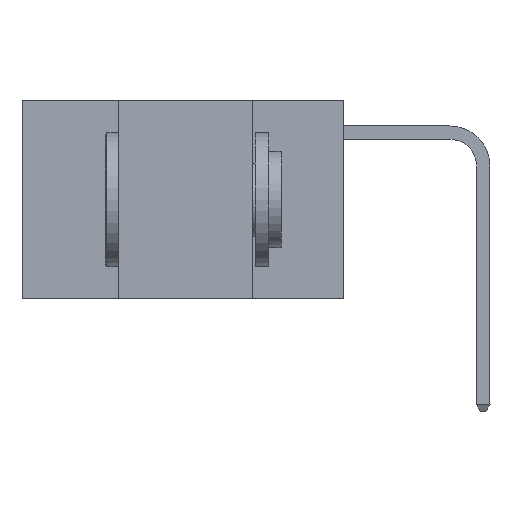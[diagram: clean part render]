
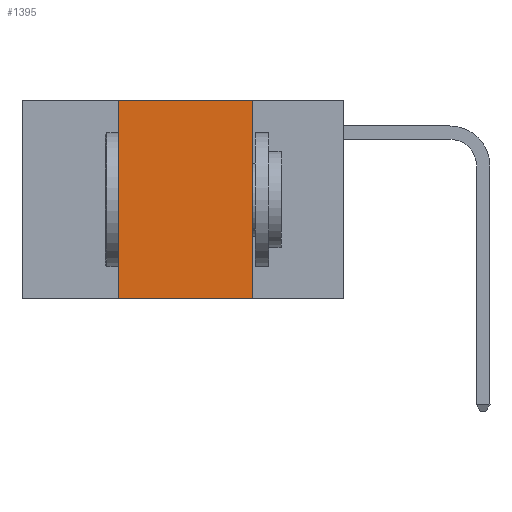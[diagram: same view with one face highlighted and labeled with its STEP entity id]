
A CAD part, left-side view. The second image highlights one B-rep face of the part: STEP entity #1395.
In plain terms, the highlighted planar face has unit normal (-1, 0, 0).
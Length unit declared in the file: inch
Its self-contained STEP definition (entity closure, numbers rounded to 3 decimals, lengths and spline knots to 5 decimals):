
#246 = CARTESIAN_POINT ( 'NONE',  ( 0., 0.42, -0.37 ) ) ;
#739 = ORIENTED_EDGE ( 'NONE', *, *, #8518, .F. ) ;
#756 = ORIENTED_EDGE ( 'NONE', *, *, #2793, .F. ) ;
#1099 = LINE ( 'NONE', #11558, #6491 ) ;
#1395 = ADVANCED_FACE ( 'NONE', ( #13389 ), #9598, .F. ) ;
#1751 = EDGE_LOOP ( 'NONE', ( #1821, #756, #739, #4710 ) ) ;
#1821 = ORIENTED_EDGE ( 'NONE', *, *, #4781, .F. ) ;
#2010 = DIRECTION ( 'NONE',  ( 1., 0., 0. ) ) ;
#2324 = DIRECTION ( 'NONE',  ( 0., 0., 1. ) ) ;
#2411 = VECTOR ( 'NONE', #10360, 39.37008 ) ;
#2793 = EDGE_CURVE ( 'NONE', #4568, #4338, #10934, .T. ) ;
#2833 = CARTESIAN_POINT ( 'NONE',  ( 0., 0.6, 0. ) ) ;
#3385 = VECTOR ( 'NONE', #2324, 39.37008 ) ;
#3481 = LINE ( 'NONE', #10780, #11895 ) ;
#4338 = VERTEX_POINT ( 'NONE', #7771 ) ;
#4568 = VERTEX_POINT ( 'NONE', #12615 ) ;
#4710 = ORIENTED_EDGE ( 'NONE', *, *, #5644, .T. ) ;
#4781 = EDGE_CURVE ( 'NONE', #4338, #8259, #3481, .T. ) ;
#5265 = DIRECTION ( 'NONE',  ( 0., 0., -1. ) ) ;
#5644 = EDGE_CURVE ( 'NONE', #7839, #8259, #1099, .T. ) ;
#6240 = LINE ( 'NONE', #7686, #3385 ) ;
#6491 = VECTOR ( 'NONE', #8222, 39.37008 ) ;
#7686 = CARTESIAN_POINT ( 'NONE',  ( 0., 0.42, 0. ) ) ;
#7771 = CARTESIAN_POINT ( 'NONE',  ( 0., 0.17, 0. ) ) ;
#7839 = VERTEX_POINT ( 'NONE', #246 ) ;
#8222 = DIRECTION ( 'NONE',  ( 0., -1., 0. ) ) ;
#8257 = AXIS2_PLACEMENT_3D ( 'NONE', #2833, #2010, #5265 ) ;
#8259 = VERTEX_POINT ( 'NONE', #10843 ) ;
#8518 = EDGE_CURVE ( 'NONE', #7839, #4568, #6240, .T. ) ;
#9598 = PLANE ( 'NONE',  #8257 ) ;
#10360 = DIRECTION ( 'NONE',  ( 0., -1., 0. ) ) ;
#10780 = CARTESIAN_POINT ( 'NONE',  ( 0., 0.17, 0. ) ) ;
#10843 = CARTESIAN_POINT ( 'NONE',  ( 0., 0.17, -0.37 ) ) ;
#10934 = LINE ( 'NONE', #11514, #2411 ) ;
#10956 = DIRECTION ( 'NONE',  ( 0., 0., -1. ) ) ;
#11514 = CARTESIAN_POINT ( 'NONE',  ( 0., 0.6, 0. ) ) ;
#11558 = CARTESIAN_POINT ( 'NONE',  ( 0., 0.6, -0.37 ) ) ;
#11895 = VECTOR ( 'NONE', #10956, 39.37008 ) ;
#12615 = CARTESIAN_POINT ( 'NONE',  ( 0., 0.42, 0. ) ) ;
#13389 = FACE_OUTER_BOUND ( 'NONE', #1751, .T. ) ;
